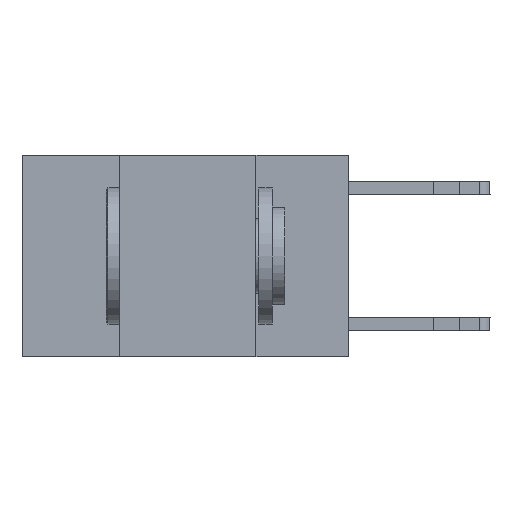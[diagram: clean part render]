
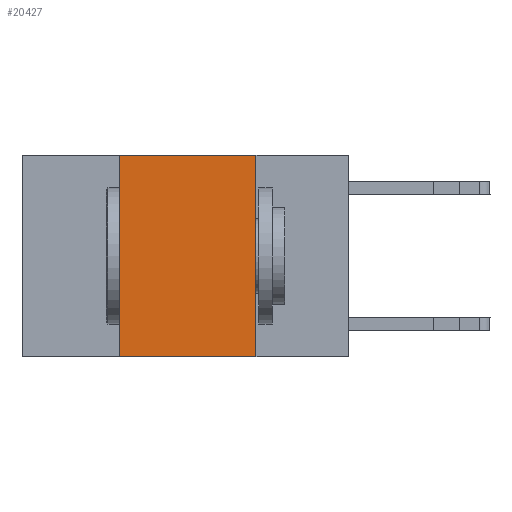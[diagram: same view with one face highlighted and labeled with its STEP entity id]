
A CAD part, left-side view. The second image highlights one B-rep face of the part: STEP entity #20427.
In plain terms, the highlighted planar face has unit normal (-1, 0, 0).
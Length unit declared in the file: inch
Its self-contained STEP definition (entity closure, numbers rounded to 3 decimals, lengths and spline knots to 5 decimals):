
#1171 = CARTESIAN_POINT ( 'NONE',  ( 0., 0.42, 0. ) ) ;
#1637 = DIRECTION ( 'NONE',  ( 0., -1., 0. ) ) ;
#1646 = VERTEX_POINT ( 'NONE', #15131 ) ;
#2751 = VECTOR ( 'NONE', #17893, 39.37008 ) ;
#3009 = DIRECTION ( 'NONE',  ( 0., 0., 1. ) ) ;
#3281 = VERTEX_POINT ( 'NONE', #14335 ) ;
#4298 = LINE ( 'NONE', #18918, #12388 ) ;
#4634 = EDGE_CURVE ( 'NONE', #1646, #3281, #4298, .T. ) ;
#5194 = VECTOR ( 'NONE', #3009, 39.37008 ) ;
#5403 = DIRECTION ( 'NONE',  ( 1., 0., 0. ) ) ;
#6331 = EDGE_LOOP ( 'NONE', ( #18213, #17781, #14583, #13686 ) ) ;
#6627 = LINE ( 'NONE', #19472, #2751 ) ;
#7373 = EDGE_CURVE ( 'NONE', #20531, #1646, #17636, .T. ) ;
#8749 = CARTESIAN_POINT ( 'NONE',  ( 0., 0.6, 0. ) ) ;
#8858 = DIRECTION ( 'NONE',  ( 0., 0., -1. ) ) ;
#9326 = LINE ( 'NONE', #15645, #5194 ) ;
#10700 = DIRECTION ( 'NONE',  ( 0., 0., -1. ) ) ;
#11512 = CARTESIAN_POINT ( 'NONE',  ( 0., 0.6, 0. ) ) ;
#12036 = EDGE_CURVE ( 'NONE', #16052, #3281, #6627, .T. ) ;
#12117 = PLANE ( 'NONE',  #14565 ) ;
#12388 = VECTOR ( 'NONE', #10700, 39.37008 ) ;
#13686 = ORIENTED_EDGE ( 'NONE', *, *, #12036, .T. ) ;
#14335 = CARTESIAN_POINT ( 'NONE',  ( 0., 0.17, -0.37 ) ) ;
#14565 = AXIS2_PLACEMENT_3D ( 'NONE', #8749, #5403, #8858 ) ;
#14583 = ORIENTED_EDGE ( 'NONE', *, *, #14731, .F. ) ;
#14731 = EDGE_CURVE ( 'NONE', #16052, #20531, #9326, .T. ) ;
#15131 = CARTESIAN_POINT ( 'NONE',  ( 0., 0.17, 0. ) ) ;
#15645 = CARTESIAN_POINT ( 'NONE',  ( 0., 0.42, 0. ) ) ;
#15791 = VECTOR ( 'NONE', #1637, 39.37008 ) ;
#16052 = VERTEX_POINT ( 'NONE', #16159 ) ;
#16159 = CARTESIAN_POINT ( 'NONE',  ( 0., 0.42, -0.37 ) ) ;
#17636 = LINE ( 'NONE', #11512, #15791 ) ;
#17781 = ORIENTED_EDGE ( 'NONE', *, *, #7373, .F. ) ;
#17893 = DIRECTION ( 'NONE',  ( 0., -1., 0. ) ) ;
#18213 = ORIENTED_EDGE ( 'NONE', *, *, #4634, .F. ) ;
#18918 = CARTESIAN_POINT ( 'NONE',  ( 0., 0.17, 0. ) ) ;
#19472 = CARTESIAN_POINT ( 'NONE',  ( 0., 0.6, -0.37 ) ) ;
#20129 = FACE_OUTER_BOUND ( 'NONE', #6331, .T. ) ;
#20427 = ADVANCED_FACE ( 'NONE', ( #20129 ), #12117, .F. ) ;
#20531 = VERTEX_POINT ( 'NONE', #1171 ) ;
